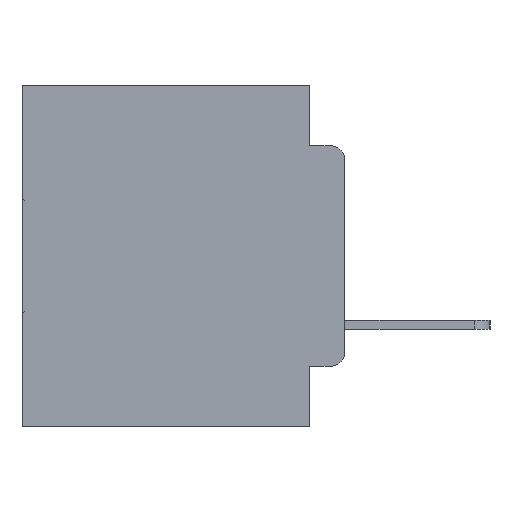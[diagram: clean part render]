
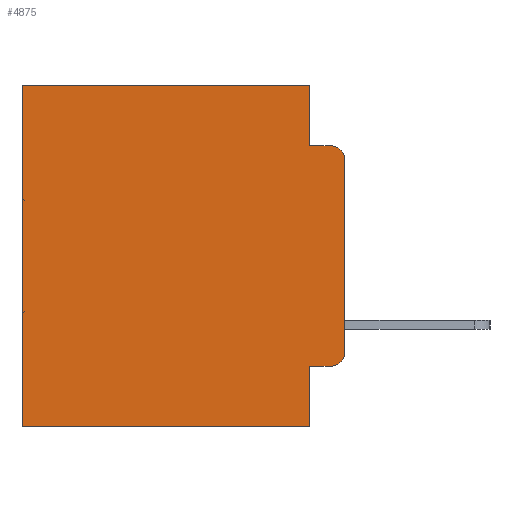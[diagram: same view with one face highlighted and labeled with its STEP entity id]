
A CAD part, left-side view. The second image highlights one B-rep face of the part: STEP entity #4875.
In plain terms, the highlighted planar face has unit normal (-1, 0, 0).
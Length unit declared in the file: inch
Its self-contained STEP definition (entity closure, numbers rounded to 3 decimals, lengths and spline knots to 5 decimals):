
#112 = VECTOR ( 'NONE', #31072, 39.37008 ) ;
#327 = EDGE_CURVE ( 'NONE', #425, #28241, #18612, .T. ) ;
#425 = VERTEX_POINT ( 'NONE', #27529 ) ;
#763 = EDGE_CURVE ( 'NONE', #20689, #2568, #5557, .T. ) ;
#1400 = CARTESIAN_POINT ( 'NONE',  ( 0.298, 0.051, -0.5 ) ) ;
#1728 = CARTESIAN_POINT ( 'NONE',  ( 0.298, 0., 0. ) ) ;
#1774 = CARTESIAN_POINT ( 'NONE',  ( 0.298, 0.051, -0.4115 ) ) ;
#2332 = EDGE_LOOP ( 'NONE', ( #29819, #16746, #17547, #19160, #6159, #13917, #20749, #8650, #23920, #22336 ) ) ;
#2568 = VERTEX_POINT ( 'NONE', #15193 ) ;
#3004 = EDGE_CURVE ( 'NONE', #22477, #18029, #6669, .T. ) ;
#4875 = ADVANCED_FACE ( 'NONE', ( #27316 ), #18231, .F. ) ;
#5400 = DIRECTION ( 'NONE',  ( 0., 1., 0. ) ) ;
#5557 = CIRCLE ( 'NONE', #24524, 0.02 ) ;
#5649 = EDGE_CURVE ( 'NONE', #9347, #27056, #31788, .T. ) ;
#6159 = ORIENTED_EDGE ( 'NONE', *, *, #3004, .T. ) ;
#6664 = VECTOR ( 'NONE', #12179, 39.37008 ) ;
#6669 = LINE ( 'NONE', #30292, #32244 ) ;
#6780 = CARTESIAN_POINT ( 'NONE',  ( 0.298, 0.473, -0.5 ) ) ;
#7281 = LINE ( 'NONE', #8663, #112 ) ;
#8328 = VERTEX_POINT ( 'NONE', #25294 ) ;
#8330 = CARTESIAN_POINT ( 'NONE',  ( 0.298, 0., -0.3915 ) ) ;
#8650 = ORIENTED_EDGE ( 'NONE', *, *, #26362, .F. ) ;
#8663 = CARTESIAN_POINT ( 'NONE',  ( 0.298, 0.051, 0. ) ) ;
#9347 = VERTEX_POINT ( 'NONE', #1400 ) ;
#10491 = CARTESIAN_POINT ( 'NONE',  ( 0.298, 0.473, 0. ) ) ;
#11419 = EDGE_CURVE ( 'NONE', #21550, #2568, #31178, .T. ) ;
#11621 = VECTOR ( 'NONE', #29718, 39.37008 ) ;
#12043 = CARTESIAN_POINT ( 'NONE',  ( 0.298, 0., -0.5 ) ) ;
#12179 = DIRECTION ( 'NONE',  ( 0., 0., -1. ) ) ;
#12283 = LINE ( 'NONE', #1774, #25858 ) ;
#12691 = AXIS2_PLACEMENT_3D ( 'NONE', #31387, #31412, #31323 ) ;
#13812 = EDGE_CURVE ( 'NONE', #22477, #21550, #7281, .T. ) ;
#13917 = ORIENTED_EDGE ( 'NONE', *, *, #18997, .T. ) ;
#14768 = CARTESIAN_POINT ( 'NONE',  ( 0.298, 0.051, 0. ) ) ;
#15135 = CARTESIAN_POINT ( 'NONE',  ( 0.298, 0., 0. ) ) ;
#15193 = CARTESIAN_POINT ( 'NONE',  ( 0.298, 0.02, -0.0885 ) ) ;
#15206 = DIRECTION ( 'NONE',  ( 0., 0., -1. ) ) ;
#16405 = CARTESIAN_POINT ( 'NONE',  ( 0.298, 0.051, 0. ) ) ;
#16638 = EDGE_CURVE ( 'NONE', #20689, #28241, #20440, .T. ) ;
#16746 = ORIENTED_EDGE ( 'NONE', *, *, #763, .T. ) ;
#17547 = ORIENTED_EDGE ( 'NONE', *, *, #11419, .F. ) ;
#18029 = VERTEX_POINT ( 'NONE', #10491 ) ;
#18189 = DIRECTION ( 'NONE',  ( 1., 0., 0. ) ) ;
#18231 = PLANE ( 'NONE',  #27239 ) ;
#18501 = LINE ( 'NONE', #14768, #11621 ) ;
#18612 = CIRCLE ( 'NONE', #12691, 0.02 ) ;
#18997 = EDGE_CURVE ( 'NONE', #18029, #27056, #32205, .T. ) ;
#19081 = VECTOR ( 'NONE', #5400, 39.37008 ) ;
#19160 = ORIENTED_EDGE ( 'NONE', *, *, #13812, .F. ) ;
#20026 = DIRECTION ( 'NONE',  ( 0., -1., 0. ) ) ;
#20235 = DIRECTION ( 'NONE',  ( 0., 0., -1. ) ) ;
#20266 = DIRECTION ( 'NONE',  ( -1., 0., 0. ) ) ;
#20440 = LINE ( 'NONE', #1728, #6664 ) ;
#20689 = VERTEX_POINT ( 'NONE', #30889 ) ;
#20749 = ORIENTED_EDGE ( 'NONE', *, *, #5649, .F. ) ;
#21167 = VECTOR ( 'NONE', #22217, 39.37008 ) ;
#21550 = VERTEX_POINT ( 'NONE', #22471 ) ;
#21737 = CARTESIAN_POINT ( 'NONE',  ( 0.298, 0.02, -0.1085 ) ) ;
#22217 = DIRECTION ( 'NONE',  ( 0., 0., -1. ) ) ;
#22336 = ORIENTED_EDGE ( 'NONE', *, *, #327, .T. ) ;
#22471 = CARTESIAN_POINT ( 'NONE',  ( 0.298, 0.051, -0.0885 ) ) ;
#22477 = VERTEX_POINT ( 'NONE', #16405 ) ;
#23920 = ORIENTED_EDGE ( 'NONE', *, *, #32318, .T. ) ;
#24524 = AXIS2_PLACEMENT_3D ( 'NONE', #21737, #20266, #20235 ) ;
#25061 = VECTOR ( 'NONE', #30548, 39.37008 ) ;
#25294 = CARTESIAN_POINT ( 'NONE',  ( 0.298, 0.051, -0.4115 ) ) ;
#25858 = VECTOR ( 'NONE', #20026, 39.37008 ) ;
#26362 = EDGE_CURVE ( 'NONE', #8328, #9347, #18501, .T. ) ;
#27056 = VERTEX_POINT ( 'NONE', #6780 ) ;
#27239 = AXIS2_PLACEMENT_3D ( 'NONE', #15135, #18189, #15206 ) ;
#27316 = FACE_OUTER_BOUND ( 'NONE', #2332, .T. ) ;
#27529 = CARTESIAN_POINT ( 'NONE',  ( 0.298, 0.02, -0.4115 ) ) ;
#28241 = VERTEX_POINT ( 'NONE', #8330 ) ;
#29488 = CARTESIAN_POINT ( 'NONE',  ( 0.298, 0.473, 0. ) ) ;
#29718 = DIRECTION ( 'NONE',  ( 0., 0., -1. ) ) ;
#29819 = ORIENTED_EDGE ( 'NONE', *, *, #16638, .F. ) ;
#30227 = DIRECTION ( 'NONE',  ( 0., 1., 0. ) ) ;
#30292 = CARTESIAN_POINT ( 'NONE',  ( 0.298, 0., 0. ) ) ;
#30548 = DIRECTION ( 'NONE',  ( 0., -1., 0. ) ) ;
#30889 = CARTESIAN_POINT ( 'NONE',  ( 0.298, 0., -0.1085 ) ) ;
#31072 = DIRECTION ( 'NONE',  ( 0., 0., -1. ) ) ;
#31178 = LINE ( 'NONE', #31280, #25061 ) ;
#31280 = CARTESIAN_POINT ( 'NONE',  ( 0.298, 0.051, -0.0885 ) ) ;
#31323 = DIRECTION ( 'NONE',  ( 0., 0., -1. ) ) ;
#31387 = CARTESIAN_POINT ( 'NONE',  ( 0.298, 0.02, -0.3915 ) ) ;
#31412 = DIRECTION ( 'NONE',  ( -1., 0., 0. ) ) ;
#31788 = LINE ( 'NONE', #12043, #19081 ) ;
#32205 = LINE ( 'NONE', #29488, #21167 ) ;
#32244 = VECTOR ( 'NONE', #30227, 39.37008 ) ;
#32318 = EDGE_CURVE ( 'NONE', #8328, #425, #12283, .T. ) ;
